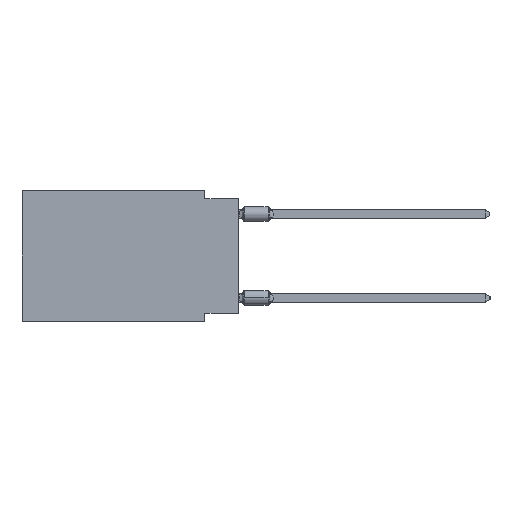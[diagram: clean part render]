
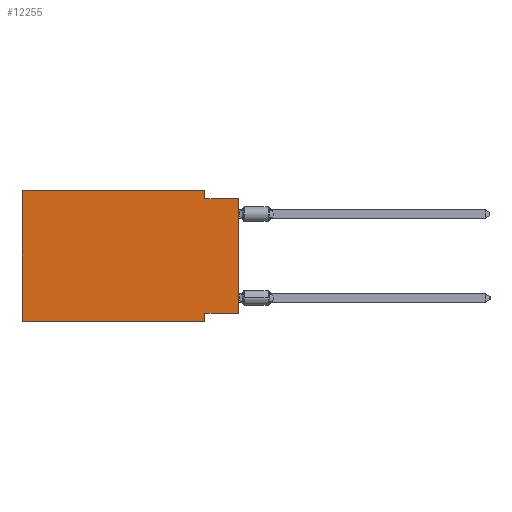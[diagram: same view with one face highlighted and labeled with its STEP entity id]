
A CAD part, left-side view. The second image highlights one B-rep face of the part: STEP entity #12255.
In plain terms, the highlighted planar face has unit normal (-1, 0, 0).
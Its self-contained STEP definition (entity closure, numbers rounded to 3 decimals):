
#290 = VECTOR ( 'NONE', #23908, 1000. ) ;
#680 = VERTEX_POINT ( 'NONE', #46702 ) ;
#1246 = LINE ( 'NONE', #16450, #34873 ) ;
#1621 = EDGE_CURVE ( 'NONE', #12939, #680, #28064, .T. ) ;
#1757 = EDGE_CURVE ( 'NONE', #680, #35452, #44336, .T. ) ;
#1784 = LINE ( 'NONE', #40010, #31958 ) ;
#1825 = CARTESIAN_POINT ( 'NONE',  ( 0., 16.383, 0. ) ) ;
#2002 = DIRECTION ( 'NONE',  ( 0., 0., -1. ) ) ;
#2852 = CARTESIAN_POINT ( 'NONE',  ( 0., 2.54, -9.906 ) ) ;
#2955 = ORIENTED_EDGE ( 'NONE', *, *, #1621, .F. ) ;
#4552 = PLANE ( 'NONE',  #21198 ) ;
#4586 = EDGE_CURVE ( 'NONE', #22840, #35452, #32368, .T. ) ;
#5876 = CARTESIAN_POINT ( 'NONE',  ( 0., 16.383, -9.906 ) ) ;
#6834 = DIRECTION ( 'NONE',  ( 0., 0., -1. ) ) ;
#7167 = VECTOR ( 'NONE', #15871, 1000. ) ;
#7298 = EDGE_CURVE ( 'NONE', #27571, #10354, #29537, .T. ) ;
#7632 = CARTESIAN_POINT ( 'NONE',  ( 0., 0., -9.271 ) ) ;
#7635 = EDGE_CURVE ( 'NONE', #10354, #33929, #1246, .T. ) ;
#8075 = VECTOR ( 'NONE', #6834, 1000. ) ;
#8671 = LINE ( 'NONE', #16152, #290 ) ;
#9825 = CARTESIAN_POINT ( 'NONE',  ( 0., 2.54, -9.906 ) ) ;
#10120 = CARTESIAN_POINT ( 'NONE',  ( 0., 2.54, -0.635 ) ) ;
#10283 = DIRECTION ( 'NONE',  ( 0., -1., 0. ) ) ;
#10354 = VERTEX_POINT ( 'NONE', #21385 ) ;
#11544 = DIRECTION ( 'NONE',  ( 0., 0., -1. ) ) ;
#12255 = ADVANCED_FACE ( 'NONE', ( #31043 ), #4552, .F. ) ;
#12374 = LINE ( 'NONE', #23381, #7167 ) ;
#12939 = VERTEX_POINT ( 'NONE', #7632 ) ;
#15234 = VECTOR ( 'NONE', #23816, 1000. ) ;
#15871 = DIRECTION ( 'NONE',  ( 0., 0., 1. ) ) ;
#16152 = CARTESIAN_POINT ( 'NONE',  ( 0., 0., -0.635 ) ) ;
#16450 = CARTESIAN_POINT ( 'NONE',  ( 0., 2.54, 0. ) ) ;
#17883 = VERTEX_POINT ( 'NONE', #47050 ) ;
#18683 = VECTOR ( 'NONE', #36363, 1000. ) ;
#19772 = CARTESIAN_POINT ( 'NONE',  ( 0., 16.383, 0. ) ) ;
#21198 = AXIS2_PLACEMENT_3D ( 'NONE', #19772, #22800, #11544 ) ;
#21385 = CARTESIAN_POINT ( 'NONE',  ( 0., 2.54, 0. ) ) ;
#21564 = EDGE_CURVE ( 'NONE', #22840, #27571, #12374, .T. ) ;
#22800 = DIRECTION ( 'NONE',  ( 1., 0., 0. ) ) ;
#22840 = VERTEX_POINT ( 'NONE', #37598 ) ;
#23381 = CARTESIAN_POINT ( 'NONE',  ( 0., 16.383, 0. ) ) ;
#23816 = DIRECTION ( 'NONE',  ( 0., 1., 0. ) ) ;
#23908 = DIRECTION ( 'NONE',  ( 0., -1., 0. ) ) ;
#24717 = EDGE_CURVE ( 'NONE', #12939, #17883, #1784, .T. ) ;
#24817 = CARTESIAN_POINT ( 'NONE',  ( 0., 0., -9.271 ) ) ;
#27571 = VERTEX_POINT ( 'NONE', #1825 ) ;
#27997 = ORIENTED_EDGE ( 'NONE', *, *, #7298, .F. ) ;
#28064 = LINE ( 'NONE', #24817, #15234 ) ;
#29537 = LINE ( 'NONE', #40808, #40478 ) ;
#31043 = FACE_OUTER_BOUND ( 'NONE', #43361, .T. ) ;
#31958 = VECTOR ( 'NONE', #39266, 1000. ) ;
#32368 = LINE ( 'NONE', #5876, #18683 ) ;
#33929 = VERTEX_POINT ( 'NONE', #10120 ) ;
#34873 = VECTOR ( 'NONE', #2002, 1000. ) ;
#35452 = VERTEX_POINT ( 'NONE', #9825 ) ;
#36315 = ORIENTED_EDGE ( 'NONE', *, *, #42525, .F. ) ;
#36363 = DIRECTION ( 'NONE',  ( 0., -1., 0. ) ) ;
#37065 = ORIENTED_EDGE ( 'NONE', *, *, #7635, .F. ) ;
#37257 = ORIENTED_EDGE ( 'NONE', *, *, #21564, .F. ) ;
#37598 = CARTESIAN_POINT ( 'NONE',  ( 0., 16.383, -9.906 ) ) ;
#37636 = ORIENTED_EDGE ( 'NONE', *, *, #24717, .T. ) ;
#39266 = DIRECTION ( 'NONE',  ( 0., 0., 1. ) ) ;
#40010 = CARTESIAN_POINT ( 'NONE',  ( 0., 0., 0. ) ) ;
#40478 = VECTOR ( 'NONE', #10283, 1000. ) ;
#40634 = ORIENTED_EDGE ( 'NONE', *, *, #1757, .F. ) ;
#40808 = CARTESIAN_POINT ( 'NONE',  ( 0., 16.383, 0. ) ) ;
#42525 = EDGE_CURVE ( 'NONE', #33929, #17883, #8671, .T. ) ;
#43361 = EDGE_LOOP ( 'NONE', ( #37636, #36315, #37065, #27997, #37257, #49076, #40634, #2955 ) ) ;
#44336 = LINE ( 'NONE', #2852, #8075 ) ;
#46702 = CARTESIAN_POINT ( 'NONE',  ( 0., 2.54, -9.271 ) ) ;
#47050 = CARTESIAN_POINT ( 'NONE',  ( 0., 0., -0.635 ) ) ;
#49076 = ORIENTED_EDGE ( 'NONE', *, *, #4586, .T. ) ;
